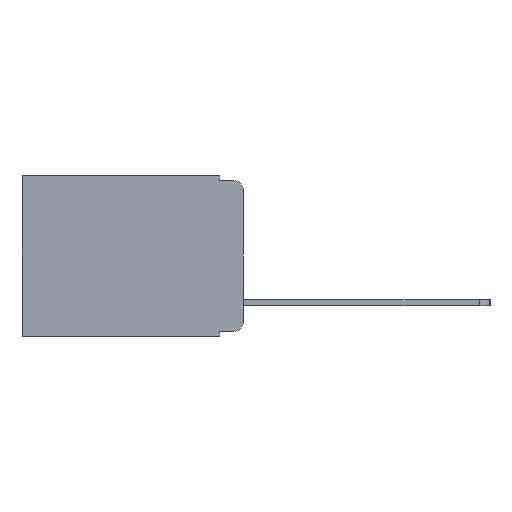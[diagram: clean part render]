
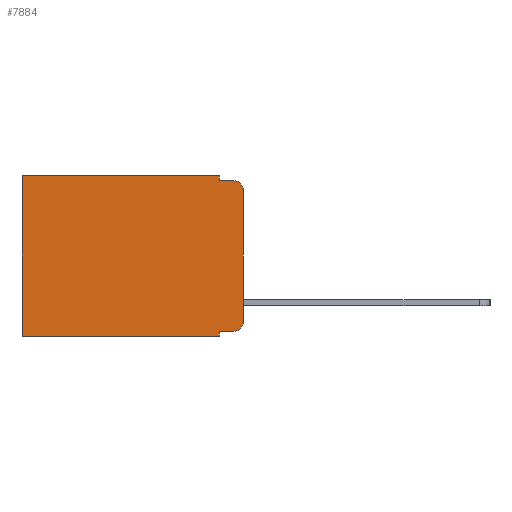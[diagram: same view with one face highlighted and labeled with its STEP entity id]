
A CAD part, left-side view. The second image highlights one B-rep face of the part: STEP entity #7884.
In plain terms, the highlighted planar face has unit normal (-1, 0, 0).
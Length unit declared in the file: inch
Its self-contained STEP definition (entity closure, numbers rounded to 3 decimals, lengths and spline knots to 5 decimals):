
#446 = CARTESIAN_POINT ( 'NONE',  ( 0.298, 0.02, -0.01 ) ) ;
#904 = EDGE_CURVE ( 'NONE', #9660, #7503, #17756, .T. ) ;
#1021 = ORIENTED_EDGE ( 'NONE', *, *, #19314, .T. ) ;
#1514 = CARTESIAN_POINT ( 'NONE',  ( 0.298, 0., 0. ) ) ;
#1847 = VECTOR ( 'NONE', #21393, 39.37008 ) ;
#2146 = CARTESIAN_POINT ( 'NONE',  ( 0.298, 0., 0. ) ) ;
#2207 = EDGE_CURVE ( 'NONE', #4120, #7503, #15013, .T. ) ;
#2464 = LINE ( 'NONE', #19701, #1847 ) ;
#2608 = VECTOR ( 'NONE', #9324, 39.37008 ) ;
#2872 = VERTEX_POINT ( 'NONE', #6525 ) ;
#2877 = VERTEX_POINT ( 'NONE', #13578 ) ;
#3183 = LINE ( 'NONE', #12881, #2608 ) ;
#3263 = DIRECTION ( 'NONE',  ( 0., 0., -1. ) ) ;
#3414 = CARTESIAN_POINT ( 'NONE',  ( 0.298, 0.051, -0.01 ) ) ;
#3426 = DIRECTION ( 'NONE',  ( 0., 0., -1. ) ) ;
#3594 = VERTEX_POINT ( 'NONE', #22547 ) ;
#4120 = VERTEX_POINT ( 'NONE', #17353 ) ;
#4654 = VERTEX_POINT ( 'NONE', #15542 ) ;
#4683 = VECTOR ( 'NONE', #3263, 39.37008 ) ;
#4865 = DIRECTION ( 'NONE',  ( 0., 0., -1. ) ) ;
#4872 = ORIENTED_EDGE ( 'NONE', *, *, #21568, .T. ) ;
#5401 = CARTESIAN_POINT ( 'NONE',  ( 0.298, 0.051, 0. ) ) ;
#5979 = EDGE_CURVE ( 'NONE', #4120, #4654, #17154, .T. ) ;
#6049 = ORIENTED_EDGE ( 'NONE', *, *, #18178, .T. ) ;
#6525 = CARTESIAN_POINT ( 'NONE',  ( 0.298, 0.051, -0.343 ) ) ;
#6740 = EDGE_CURVE ( 'NONE', #2872, #16894, #3183, .T. ) ;
#6978 = VECTOR ( 'NONE', #20271, 39.37008 ) ;
#7069 = CARTESIAN_POINT ( 'NONE',  ( 0.298, 0.473, 0. ) ) ;
#7398 = CARTESIAN_POINT ( 'NONE',  ( 0.298, 0., 0. ) ) ;
#7503 = VERTEX_POINT ( 'NONE', #446 ) ;
#7770 = ORIENTED_EDGE ( 'NONE', *, *, #2207, .T. ) ;
#7884 = ADVANCED_FACE ( 'NONE', ( #8311 ), #10626, .F. ) ;
#8041 = DIRECTION ( 'NONE',  ( -1., 0., 0. ) ) ;
#8311 = FACE_OUTER_BOUND ( 'NONE', #9685, .T. ) ;
#8585 = ORIENTED_EDGE ( 'NONE', *, *, #18042, .T. ) ;
#8727 = VECTOR ( 'NONE', #10776, 39.37008 ) ;
#9324 = DIRECTION ( 'NONE',  ( 0., 1., 0. ) ) ;
#9426 = DIRECTION ( 'NONE',  ( -1., 0., 0. ) ) ;
#9509 = CARTESIAN_POINT ( 'NONE',  ( 0.298, 0.02, -0.03 ) ) ;
#9517 = LINE ( 'NONE', #15782, #4683 ) ;
#9660 = VERTEX_POINT ( 'NONE', #12330 ) ;
#9685 = EDGE_LOOP ( 'NONE', ( #21054, #7770, #17088, #21585, #8585, #4872, #9697, #14349, #1021, #6049 ) ) ;
#9697 = ORIENTED_EDGE ( 'NONE', *, *, #6740, .F. ) ;
#10626 = PLANE ( 'NONE',  #15626 ) ;
#10776 = DIRECTION ( 'NONE',  ( 0., 0., -1. ) ) ;
#11033 = CARTESIAN_POINT ( 'NONE',  ( 0.298, 0.473, -0.343 ) ) ;
#11271 = DIRECTION ( 'NONE',  ( 0., -1., 0. ) ) ;
#12233 = LINE ( 'NONE', #18573, #6978 ) ;
#12330 = CARTESIAN_POINT ( 'NONE',  ( 0.298, 0.051, -0.01 ) ) ;
#12600 = VERTEX_POINT ( 'NONE', #17665 ) ;
#12881 = CARTESIAN_POINT ( 'NONE',  ( 0.298, 0., -0.343 ) ) ;
#13425 = LINE ( 'NONE', #5401, #8727 ) ;
#13578 = CARTESIAN_POINT ( 'NONE',  ( 0.298, 0.02, -0.333 ) ) ;
#14066 = LINE ( 'NONE', #2146, #22081 ) ;
#14177 = DIRECTION ( 'NONE',  ( 1., 0., 0. ) ) ;
#14349 = ORIENTED_EDGE ( 'NONE', *, *, #20441, .F. ) ;
#14486 = DIRECTION ( 'NONE',  ( 0., 0., -1. ) ) ;
#14648 = AXIS2_PLACEMENT_3D ( 'NONE', #9509, #9426, #4865 ) ;
#15013 = CIRCLE ( 'NONE', #14648, 0.02 ) ;
#15542 = CARTESIAN_POINT ( 'NONE',  ( 0.298, 0., -0.313 ) ) ;
#15626 = AXIS2_PLACEMENT_3D ( 'NONE', #1514, #14177, #3426 ) ;
#15782 = CARTESIAN_POINT ( 'NONE',  ( 0.298, 0.473, 0. ) ) ;
#15971 = CIRCLE ( 'NONE', #19935, 0.02 ) ;
#16894 = VERTEX_POINT ( 'NONE', #11033 ) ;
#17088 = ORIENTED_EDGE ( 'NONE', *, *, #904, .F. ) ;
#17154 = LINE ( 'NONE', #7398, #21653 ) ;
#17234 = VECTOR ( 'NONE', #11271, 39.37008 ) ;
#17353 = CARTESIAN_POINT ( 'NONE',  ( 0.298, 0., -0.03 ) ) ;
#17665 = CARTESIAN_POINT ( 'NONE',  ( 0.298, 0.051, -0.333 ) ) ;
#17756 = LINE ( 'NONE', #3414, #17234 ) ;
#18042 = EDGE_CURVE ( 'NONE', #3594, #21627, #14066, .T. ) ;
#18178 = EDGE_CURVE ( 'NONE', #2877, #4654, #15971, .T. ) ;
#18192 = DIRECTION ( 'NONE',  ( 0., 1., 0. ) ) ;
#18493 = CARTESIAN_POINT ( 'NONE',  ( 0.298, 0.02, -0.313 ) ) ;
#18573 = CARTESIAN_POINT ( 'NONE',  ( 0.298, 0.051, 0. ) ) ;
#19314 = EDGE_CURVE ( 'NONE', #12600, #2877, #2464, .T. ) ;
#19701 = CARTESIAN_POINT ( 'NONE',  ( 0.298, 0.051, -0.333 ) ) ;
#19935 = AXIS2_PLACEMENT_3D ( 'NONE', #18493, #8041, #20182 ) ;
#20182 = DIRECTION ( 'NONE',  ( 0., 0., -1. ) ) ;
#20271 = DIRECTION ( 'NONE',  ( 0., 0., -1. ) ) ;
#20441 = EDGE_CURVE ( 'NONE', #12600, #2872, #13425, .T. ) ;
#21054 = ORIENTED_EDGE ( 'NONE', *, *, #5979, .F. ) ;
#21393 = DIRECTION ( 'NONE',  ( 0., -1., 0. ) ) ;
#21568 = EDGE_CURVE ( 'NONE', #21627, #16894, #9517, .T. ) ;
#21585 = ORIENTED_EDGE ( 'NONE', *, *, #22694, .F. ) ;
#21627 = VERTEX_POINT ( 'NONE', #7069 ) ;
#21653 = VECTOR ( 'NONE', #14486, 39.37008 ) ;
#22081 = VECTOR ( 'NONE', #18192, 39.37008 ) ;
#22547 = CARTESIAN_POINT ( 'NONE',  ( 0.298, 0.051, 0. ) ) ;
#22694 = EDGE_CURVE ( 'NONE', #3594, #9660, #12233, .T. ) ;
